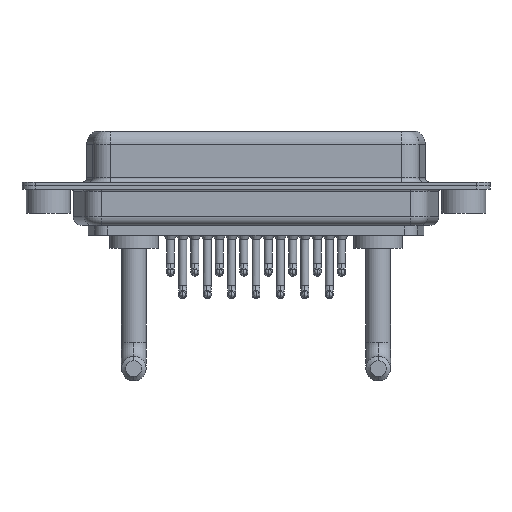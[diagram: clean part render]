
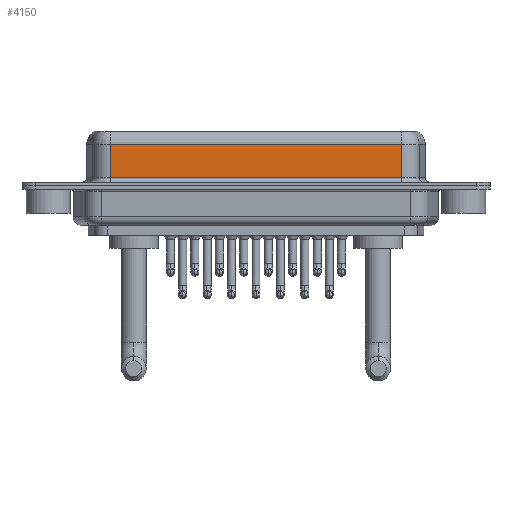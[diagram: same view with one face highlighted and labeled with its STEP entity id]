
A CAD part, front view. The second image highlights one B-rep face of the part: STEP entity #4150.
In plain terms, the highlighted planar face has unit normal (0, -1, 0).
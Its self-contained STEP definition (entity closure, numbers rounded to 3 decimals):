
#999 = LINE ( 'NONE', #4380, #4133 ) ;
#1314 = DIRECTION ( 'NONE',  ( 0., 0., -1. ) ) ;
#2668 = CARTESIAN_POINT ( 'NONE',  ( 7.013, -3.95, 0.9 ) ) ;
#2962 = LINE ( 'NONE', #20250, #13633 ) ;
#3804 = ORIENTED_EDGE ( 'NONE', *, *, #3992, .F. ) ;
#3992 = EDGE_CURVE ( 'NONE', #5719, #4188, #12094, .T. ) ;
#4133 = VECTOR ( 'NONE', #1314, 1000. ) ;
#4150 = ADVANCED_FACE ( 'NONE', ( #19142 ), #15779, .F. ) ;
#4188 = VERTEX_POINT ( 'NONE', #4711 ) ;
#4233 = DIRECTION ( 'NONE',  ( -1., 0., 0. ) ) ;
#4380 = CARTESIAN_POINT ( 'NONE',  ( 7.013, -3.95, 6.4 ) ) ;
#4711 = CARTESIAN_POINT ( 'NONE',  ( 40.037, -3.95, 0.9 ) ) ;
#5719 = VERTEX_POINT ( 'NONE', #13238 ) ;
#5871 = CARTESIAN_POINT ( 'NONE',  ( 40.037, -3.95, 6.4 ) ) ;
#6590 = EDGE_CURVE ( 'NONE', #11875, #15524, #999, .T. ) ;
#7862 = CARTESIAN_POINT ( 'NONE',  ( 7.013, -3.95, 4.65 ) ) ;
#8335 = EDGE_LOOP ( 'NONE', ( #3804, #14987, #14694, #18359 ) ) ;
#9224 = EDGE_CURVE ( 'NONE', #5719, #11875, #2962, .T. ) ;
#9866 = EDGE_CURVE ( 'NONE', #15524, #4188, #19755, .T. ) ;
#10534 = DIRECTION ( 'NONE',  ( 0., 0., -1. ) ) ;
#11030 = DIRECTION ( 'NONE',  ( 0., 0., 1. ) ) ;
#11875 = VERTEX_POINT ( 'NONE', #7862 ) ;
#12094 = LINE ( 'NONE', #5871, #13655 ) ;
#12498 = CARTESIAN_POINT ( 'NONE',  ( 40.037, -3.95, 6.4 ) ) ;
#13238 = CARTESIAN_POINT ( 'NONE',  ( 40.037, -3.95, 4.65 ) ) ;
#13633 = VECTOR ( 'NONE', #4233, 1000. ) ;
#13655 = VECTOR ( 'NONE', #10534, 1000. ) ;
#14693 = AXIS2_PLACEMENT_3D ( 'NONE', #12498, #20505, #11030 ) ;
#14694 = ORIENTED_EDGE ( 'NONE', *, *, #6590, .T. ) ;
#14987 = ORIENTED_EDGE ( 'NONE', *, *, #9224, .T. ) ;
#15524 = VERTEX_POINT ( 'NONE', #2668 ) ;
#15779 = PLANE ( 'NONE',  #14693 ) ;
#15982 = VECTOR ( 'NONE', #18182, 1000. ) ;
#16289 = CARTESIAN_POINT ( 'NONE',  ( 40.037, -3.95, 0.9 ) ) ;
#18182 = DIRECTION ( 'NONE',  ( 1., 0., 0. ) ) ;
#18359 = ORIENTED_EDGE ( 'NONE', *, *, #9866, .T. ) ;
#19142 = FACE_OUTER_BOUND ( 'NONE', #8335, .T. ) ;
#19755 = LINE ( 'NONE', #16289, #15982 ) ;
#20250 = CARTESIAN_POINT ( 'NONE',  ( 40.037, -3.95, 4.65 ) ) ;
#20505 = DIRECTION ( 'NONE',  ( 0., 1., 0. ) ) ;
